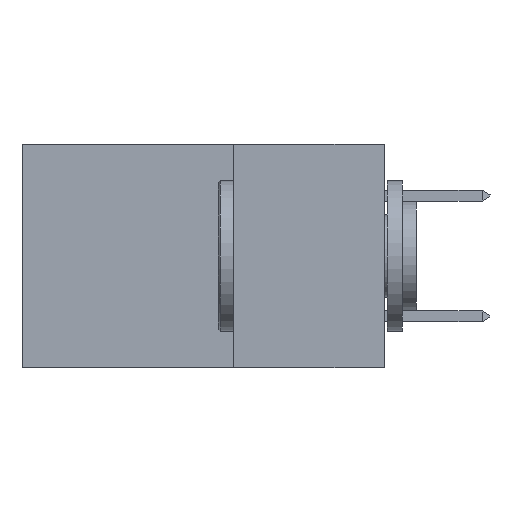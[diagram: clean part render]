
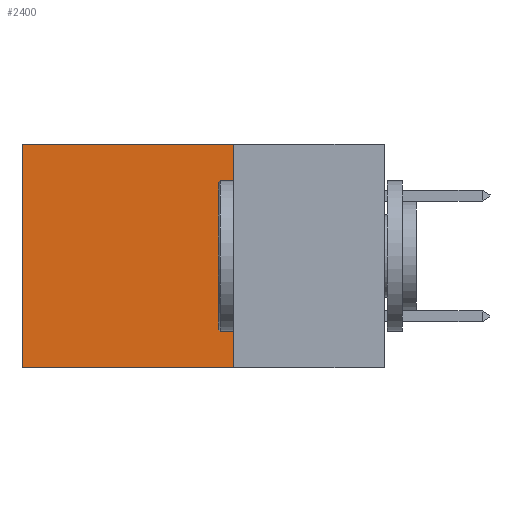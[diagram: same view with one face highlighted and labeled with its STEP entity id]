
A CAD part, left-side view. The second image highlights one B-rep face of the part: STEP entity #2400.
In plain terms, the highlighted planar face has unit normal (-1, 0, 0).
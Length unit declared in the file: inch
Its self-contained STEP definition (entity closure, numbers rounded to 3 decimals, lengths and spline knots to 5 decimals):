
#249 = VERTEX_POINT ( 'NONE', #16853 ) ;
#562 = CARTESIAN_POINT ( 'NONE',  ( 0.2875, 0.25, 0. ) ) ;
#1614 = VERTEX_POINT ( 'NONE', #3939 ) ;
#2400 = ADVANCED_FACE ( 'NONE', ( #3411 ), #21600, .F. ) ;
#3179 = ORIENTED_EDGE ( 'NONE', *, *, #21262, .F. ) ;
#3411 = FACE_OUTER_BOUND ( 'NONE', #9356, .T. ) ;
#3939 = CARTESIAN_POINT ( 'NONE',  ( 0.2875, 0.6, -0.37 ) ) ;
#4106 = DIRECTION ( 'NONE',  ( 0., 1., 0. ) ) ;
#4186 = CARTESIAN_POINT ( 'NONE',  ( 0.2875, 0.25, -0.37 ) ) ;
#6591 = ORIENTED_EDGE ( 'NONE', *, *, #13656, .F. ) ;
#6933 = VERTEX_POINT ( 'NONE', #4186 ) ;
#7538 = DIRECTION ( 'NONE',  ( 1., 0., 0. ) ) ;
#8047 = CARTESIAN_POINT ( 'NONE',  ( 0.2875, 0.6, 0. ) ) ;
#9356 = EDGE_LOOP ( 'NONE', ( #29651, #3179, #6591, #10117 ) ) ;
#10117 = ORIENTED_EDGE ( 'NONE', *, *, #28738, .T. ) ;
#13265 = CARTESIAN_POINT ( 'NONE',  ( 0.2875, 0.25, -0.37 ) ) ;
#13590 = VECTOR ( 'NONE', #18402, 39.37008 ) ;
#13656 = EDGE_CURVE ( 'NONE', #249, #6933, #21581, .T. ) ;
#16248 = LINE ( 'NONE', #20740, #27662 ) ;
#16853 = CARTESIAN_POINT ( 'NONE',  ( 0.2875, 0.25, 0. ) ) ;
#17643 = DIRECTION ( 'NONE',  ( 0., 0., -1. ) ) ;
#18402 = DIRECTION ( 'NONE',  ( 0., 0., -1. ) ) ;
#19440 = VECTOR ( 'NONE', #27223, 39.37008 ) ;
#20160 = LINE ( 'NONE', #13265, #19440 ) ;
#20740 = CARTESIAN_POINT ( 'NONE',  ( 0.2875, 0.25, 0. ) ) ;
#21262 = EDGE_CURVE ( 'NONE', #6933, #1614, #20160, .T. ) ;
#21581 = LINE ( 'NONE', #27780, #13590 ) ;
#21600 = PLANE ( 'NONE',  #23266 ) ;
#21721 = CARTESIAN_POINT ( 'NONE',  ( 0.2875, 0.6, 0. ) ) ;
#23266 = AXIS2_PLACEMENT_3D ( 'NONE', #562, #7538, #26400 ) ;
#25076 = VECTOR ( 'NONE', #17643, 39.37008 ) ;
#26013 = EDGE_CURVE ( 'NONE', #28361, #1614, #26188, .T. ) ;
#26188 = LINE ( 'NONE', #8047, #25076 ) ;
#26400 = DIRECTION ( 'NONE',  ( 0., 0., -1. ) ) ;
#27223 = DIRECTION ( 'NONE',  ( 0., 1., 0. ) ) ;
#27662 = VECTOR ( 'NONE', #4106, 39.37008 ) ;
#27780 = CARTESIAN_POINT ( 'NONE',  ( 0.2875, 0.25, 0. ) ) ;
#28361 = VERTEX_POINT ( 'NONE', #21721 ) ;
#28738 = EDGE_CURVE ( 'NONE', #249, #28361, #16248, .T. ) ;
#29651 = ORIENTED_EDGE ( 'NONE', *, *, #26013, .T. ) ;
